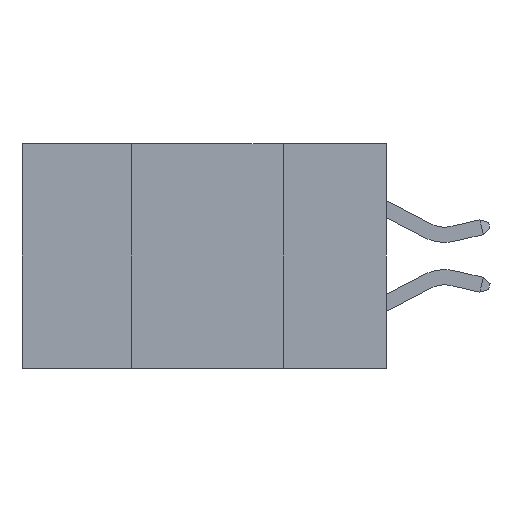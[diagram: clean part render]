
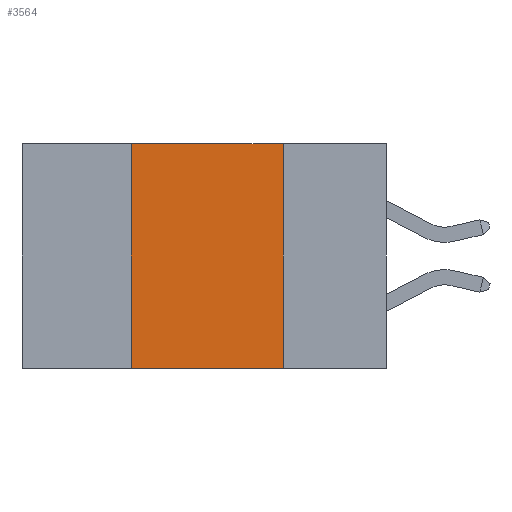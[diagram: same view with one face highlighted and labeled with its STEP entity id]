
A CAD part, left-side view. The second image highlights one B-rep face of the part: STEP entity #3564.
In plain terms, the highlighted planar face has unit normal (-1, 0, 0).
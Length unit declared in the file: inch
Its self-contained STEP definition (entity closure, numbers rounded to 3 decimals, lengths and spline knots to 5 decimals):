
#349 = VECTOR ( 'NONE', #1679, 39.37008 ) ;
#991 = CARTESIAN_POINT ( 'NONE',  ( 0., 0.42, 0. ) ) ;
#1679 = DIRECTION ( 'NONE',  ( 0., 0., -1. ) ) ;
#2284 = VERTEX_POINT ( 'NONE', #9439 ) ;
#2704 = DIRECTION ( 'NONE',  ( 0., -1., 0. ) ) ;
#3418 = EDGE_CURVE ( 'NONE', #30370, #2284, #26314, .T. ) ;
#3564 = ADVANCED_FACE ( 'NONE', ( #5665 ), #28748, .F. ) ;
#3590 = DIRECTION ( 'NONE',  ( 0., 0., -1. ) ) ;
#5665 = FACE_OUTER_BOUND ( 'NONE', #29443, .T. ) ;
#5936 = EDGE_CURVE ( 'NONE', #2284, #12460, #24187, .T. ) ;
#6066 = VECTOR ( 'NONE', #22987, 39.37008 ) ;
#6934 = VERTEX_POINT ( 'NONE', #19086 ) ;
#7766 = LINE ( 'NONE', #13992, #349 ) ;
#8198 = CARTESIAN_POINT ( 'NONE',  ( 0., 0.17, 0. ) ) ;
#9269 = ORIENTED_EDGE ( 'NONE', *, *, #3418, .F. ) ;
#9439 = CARTESIAN_POINT ( 'NONE',  ( 0., 0.42, 0. ) ) ;
#12326 = ORIENTED_EDGE ( 'NONE', *, *, #5936, .F. ) ;
#12460 = VERTEX_POINT ( 'NONE', #8198 ) ;
#13819 = CARTESIAN_POINT ( 'NONE',  ( 0., 0.6, 0. ) ) ;
#13992 = CARTESIAN_POINT ( 'NONE',  ( 0., 0.17, 0. ) ) ;
#15051 = EDGE_CURVE ( 'NONE', #12460, #6934, #7766, .T. ) ;
#16755 = EDGE_CURVE ( 'NONE', #30370, #6934, #31408, .T. ) ;
#17079 = ORIENTED_EDGE ( 'NONE', *, *, #16755, .T. ) ;
#17577 = CARTESIAN_POINT ( 'NONE',  ( 0., 0.42, -0.37 ) ) ;
#19086 = CARTESIAN_POINT ( 'NONE',  ( 0., 0.17, -0.37 ) ) ;
#21321 = VECTOR ( 'NONE', #2704, 39.37008 ) ;
#21328 = DIRECTION ( 'NONE',  ( 1., 0., 0. ) ) ;
#22415 = AXIS2_PLACEMENT_3D ( 'NONE', #13819, #21328, #3590 ) ;
#22570 = CARTESIAN_POINT ( 'NONE',  ( 0., 0.6, 0. ) ) ;
#22750 = CARTESIAN_POINT ( 'NONE',  ( 0., 0.6, -0.37 ) ) ;
#22987 = DIRECTION ( 'NONE',  ( 0., 0., 1. ) ) ;
#24187 = LINE ( 'NONE', #22570, #29264 ) ;
#26314 = LINE ( 'NONE', #991, #6066 ) ;
#28748 = PLANE ( 'NONE',  #22415 ) ;
#28848 = ORIENTED_EDGE ( 'NONE', *, *, #15051, .F. ) ;
#29264 = VECTOR ( 'NONE', #29866, 39.37008 ) ;
#29443 = EDGE_LOOP ( 'NONE', ( #28848, #12326, #9269, #17079 ) ) ;
#29866 = DIRECTION ( 'NONE',  ( 0., -1., 0. ) ) ;
#30370 = VERTEX_POINT ( 'NONE', #17577 ) ;
#31408 = LINE ( 'NONE', #22750, #21321 ) ;
